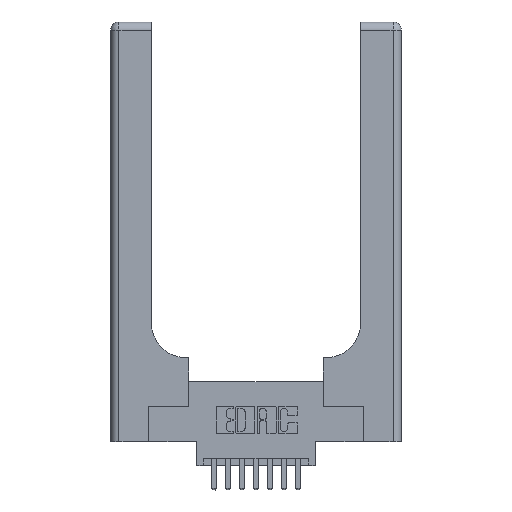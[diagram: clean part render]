
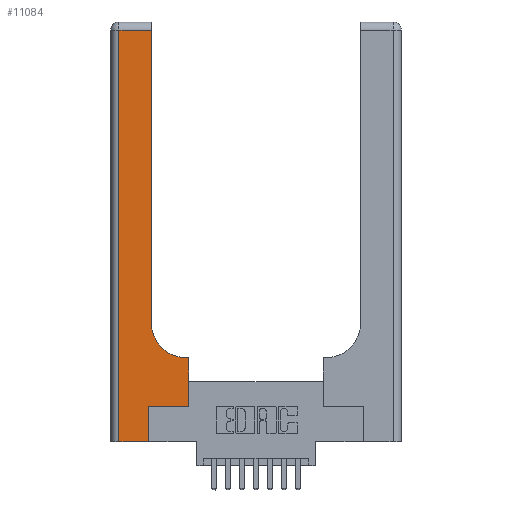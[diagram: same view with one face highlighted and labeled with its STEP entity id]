
A CAD part, top view. The second image highlights one B-rep face of the part: STEP entity #11084.
In plain terms, the highlighted planar face has unit normal (0, 0, 1).
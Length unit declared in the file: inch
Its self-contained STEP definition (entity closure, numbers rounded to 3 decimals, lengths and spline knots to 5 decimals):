
#191 = DIRECTION ( 'NONE',  ( 0., 1., 0. ) ) ;
#435 = ORIENTED_EDGE ( 'NONE', *, *, #13186, .T. ) ;
#453 = LINE ( 'NONE', #4184, #3268 ) ;
#513 = CARTESIAN_POINT ( 'NONE',  ( 0.06, 0., 0.37 ) ) ;
#519 = DIRECTION ( 'NONE',  ( 0., 1., 0. ) ) ;
#672 = EDGE_CURVE ( 'NONE', #3194, #3841, #1594, .T. ) ;
#791 = LINE ( 'NONE', #6718, #9059 ) ;
#913 = CIRCLE ( 'NONE', #14126, 0.25 ) ;
#990 = LINE ( 'NONE', #12369, #2862 ) ;
#1117 = DIRECTION ( 'NONE',  ( 0., 1., 0. ) ) ;
#1163 = VERTEX_POINT ( 'NONE', #7395 ) ;
#1594 = LINE ( 'NONE', #11239, #2514 ) ;
#1810 = EDGE_LOOP ( 'NONE', ( #3925, #2143, #7578, #7393, #435, #6135, #9941, #4124, #4782 ) ) ;
#2143 = ORIENTED_EDGE ( 'NONE', *, *, #7350, .T. ) ;
#2514 = VECTOR ( 'NONE', #191, 39.37008 ) ;
#2545 = EDGE_CURVE ( 'NONE', #14286, #4080, #791, .T. ) ;
#2707 = DIRECTION ( 'NONE',  ( -1., 0., 0. ) ) ;
#2862 = VECTOR ( 'NONE', #5157, 39.37008 ) ;
#3194 = VERTEX_POINT ( 'NONE', #10456 ) ;
#3268 = VECTOR ( 'NONE', #4296, 39.37008 ) ;
#3454 = EDGE_CURVE ( 'NONE', #13893, #12225, #913, .T. ) ;
#3690 = DIRECTION ( 'NONE',  ( -1., 0., 0. ) ) ;
#3841 = VERTEX_POINT ( 'NONE', #7977 ) ;
#3925 = ORIENTED_EDGE ( 'NONE', *, *, #5630, .T. ) ;
#4080 = VERTEX_POINT ( 'NONE', #12414 ) ;
#4124 = ORIENTED_EDGE ( 'NONE', *, *, #8473, .T. ) ;
#4184 = CARTESIAN_POINT ( 'NONE',  ( 0.06, 3., 0.37 ) ) ;
#4296 = DIRECTION ( 'NONE',  ( 0., -1., 0. ) ) ;
#4782 = ORIENTED_EDGE ( 'NONE', *, *, #3454, .T. ) ;
#5157 = DIRECTION ( 'NONE',  ( 1., 0., 0. ) ) ;
#5504 = VECTOR ( 'NONE', #2707, 39.37008 ) ;
#5619 = DIRECTION ( 'NONE',  ( 0., 0., -1. ) ) ;
#5630 = EDGE_CURVE ( 'NONE', #12225, #15388, #14235, .T. ) ;
#5708 = LINE ( 'NONE', #7570, #11783 ) ;
#5737 = CARTESIAN_POINT ( 'NONE',  ( 0.5415, 0.6, 0.37 ) ) ;
#5842 = VECTOR ( 'NONE', #3690, 39.37008 ) ;
#5885 = CARTESIAN_POINT ( 'NONE',  ( 0.2915, 3., 0.37 ) ) ;
#6135 = ORIENTED_EDGE ( 'NONE', *, *, #14889, .T. ) ;
#6718 = CARTESIAN_POINT ( 'NONE',  ( 0., 0., 0.37 ) ) ;
#6957 = DIRECTION ( 'NONE',  ( 0., 0., -1. ) ) ;
#7117 = PLANE ( 'NONE',  #10886 ) ;
#7350 = EDGE_CURVE ( 'NONE', #15388, #8615, #11957, .T. ) ;
#7357 = CARTESIAN_POINT ( 'NONE',  ( 0.2915, 0.6, 0.37 ) ) ;
#7393 = ORIENTED_EDGE ( 'NONE', *, *, #2545, .T. ) ;
#7395 = CARTESIAN_POINT ( 'NONE',  ( 0.269, 0.25, 0.37 ) ) ;
#7570 = CARTESIAN_POINT ( 'NONE',  ( 0.269, 0., 0.37 ) ) ;
#7578 = ORIENTED_EDGE ( 'NONE', *, *, #12731, .T. ) ;
#7860 = CARTESIAN_POINT ( 'NONE',  ( 0.2915, 0.85, 0.37 ) ) ;
#7977 = CARTESIAN_POINT ( 'NONE',  ( 0.5585, 0.6, 0.37 ) ) ;
#8103 = DIRECTION ( 'NONE',  ( -1., 0., 0. ) ) ;
#8473 = EDGE_CURVE ( 'NONE', #3841, #13893, #12100, .T. ) ;
#8615 = VERTEX_POINT ( 'NONE', #11166 ) ;
#9059 = VECTOR ( 'NONE', #10217, 39.37008 ) ;
#9577 = CARTESIAN_POINT ( 'NONE',  ( 0., 2.94, 0.37 ) ) ;
#9607 = CARTESIAN_POINT ( 'NONE',  ( 0.2915, 2.94, 0.37 ) ) ;
#9941 = ORIENTED_EDGE ( 'NONE', *, *, #672, .T. ) ;
#10217 = DIRECTION ( 'NONE',  ( 1., 0., 0. ) ) ;
#10456 = CARTESIAN_POINT ( 'NONE',  ( 0.5585, 0.25, 0.37 ) ) ;
#10886 = AXIS2_PLACEMENT_3D ( 'NONE', #11987, #6957, #8103 ) ;
#11084 = ADVANCED_FACE ( 'NONE', ( #14645 ), #7117, .F. ) ;
#11166 = CARTESIAN_POINT ( 'NONE',  ( 0.06, 2.94, 0.37 ) ) ;
#11239 = CARTESIAN_POINT ( 'NONE',  ( 0.5585, 0.25, 0.37 ) ) ;
#11560 = CARTESIAN_POINT ( 'NONE',  ( 0.5415, 0.85, 0.37 ) ) ;
#11783 = VECTOR ( 'NONE', #519, 39.37008 ) ;
#11957 = LINE ( 'NONE', #9577, #5504 ) ;
#11987 = CARTESIAN_POINT ( 'NONE',  ( 0., 3., 0.37 ) ) ;
#12100 = LINE ( 'NONE', #7357, #5842 ) ;
#12225 = VERTEX_POINT ( 'NONE', #7860 ) ;
#12369 = CARTESIAN_POINT ( 'NONE',  ( 0.269, 0.25, 0.37 ) ) ;
#12414 = CARTESIAN_POINT ( 'NONE',  ( 0.269, 0., 0.37 ) ) ;
#12731 = EDGE_CURVE ( 'NONE', #8615, #14286, #453, .T. ) ;
#13186 = EDGE_CURVE ( 'NONE', #4080, #1163, #5708, .T. ) ;
#13284 = VECTOR ( 'NONE', #1117, 39.37008 ) ;
#13893 = VERTEX_POINT ( 'NONE', #5737 ) ;
#14126 = AXIS2_PLACEMENT_3D ( 'NONE', #11560, #5619, #15321 ) ;
#14235 = LINE ( 'NONE', #5885, #13284 ) ;
#14286 = VERTEX_POINT ( 'NONE', #513 ) ;
#14645 = FACE_OUTER_BOUND ( 'NONE', #1810, .T. ) ;
#14889 = EDGE_CURVE ( 'NONE', #1163, #3194, #990, .T. ) ;
#15321 = DIRECTION ( 'NONE',  ( 1., 0., 0. ) ) ;
#15388 = VERTEX_POINT ( 'NONE', #9607 ) ;
